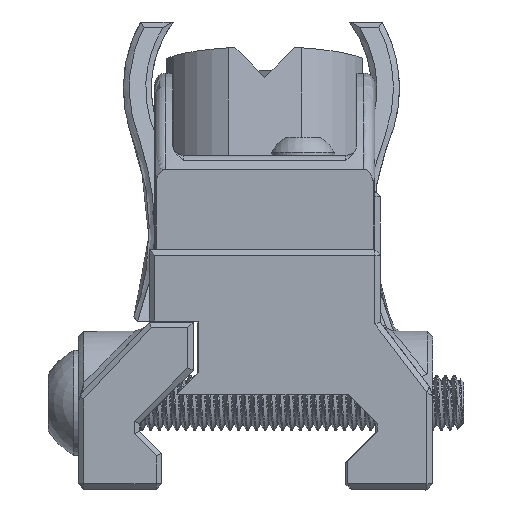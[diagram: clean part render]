
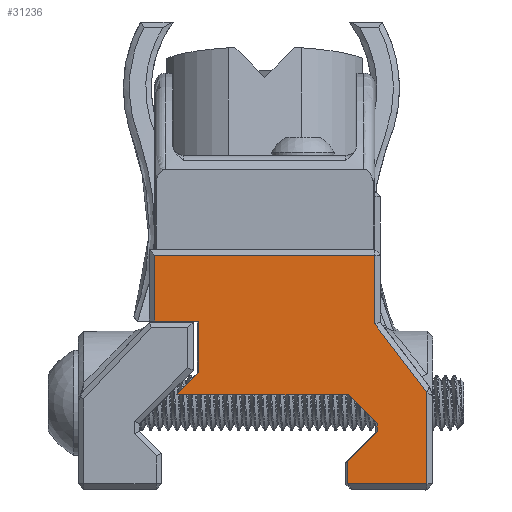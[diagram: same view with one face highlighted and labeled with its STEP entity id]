
A CAD part, front view. The second image highlights one B-rep face of the part: STEP entity #31236.
In plain terms, the highlighted planar face has unit normal (0, -1, 0).
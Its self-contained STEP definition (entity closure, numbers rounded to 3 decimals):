
#1353=PLANE('',#33986);
#4841=FACE_OUTER_BOUND('',#6821,.T.);
#6821=EDGE_LOOP('',(#26321,#26322,#26323,#26324,#26325,#26326,#26327,#26328,
#26329,#26330,#26331,#26332,#26333,#26334));
#8676=LINE('',#80153,#10592);
#8693=LINE('',#80186,#10609);
#8699=LINE('',#80198,#10615);
#8700=LINE('',#80201,#10616);
#8707=LINE('',#80217,#10623);
#8709=LINE('',#80220,#10625);
#8712=LINE('',#80224,#10628);
#8737=LINE('',#80277,#10653);
#8738=LINE('',#80279,#10654);
#8739=LINE('',#80281,#10655);
#8740=LINE('',#80283,#10656);
#8741=LINE('',#80284,#10657);
#8742=LINE('',#80286,#10658);
#8743=LINE('',#80287,#10659);
#10592=VECTOR('',#39924,10.);
#10609=VECTOR('',#39953,10.);
#10615=VECTOR('',#39967,10.);
#10616=VECTOR('',#39970,10.);
#10623=VECTOR('',#39981,10.);
#10625=VECTOR('',#39985,10.);
#10628=VECTOR('',#39990,10.);
#10653=VECTOR('',#40043,10.);
#10654=VECTOR('',#40044,10.);
#10655=VECTOR('',#40045,10.);
#10656=VECTOR('',#40046,10.);
#10657=VECTOR('',#40047,10.);
#10658=VECTOR('',#40048,10.);
#10659=VECTOR('',#40049,10.);
#14172=VERTEX_POINT('',#80150);
#14173=VERTEX_POINT('',#80152);
#14178=VERTEX_POINT('',#80167);
#14182=VERTEX_POINT('',#80179);
#14185=VERTEX_POINT('',#80194);
#14186=VERTEX_POINT('',#80200);
#14189=VERTEX_POINT('',#80207);
#14192=VERTEX_POINT('',#80214);
#14193=VERTEX_POINT('',#80216);
#14207=VERTEX_POINT('',#80276);
#14208=VERTEX_POINT('',#80278);
#14209=VERTEX_POINT('',#80280);
#14210=VERTEX_POINT('',#80282);
#14211=VERTEX_POINT('',#80285);
#18333=EDGE_CURVE('',#14172,#14173,#8676,.T.);
#18350=EDGE_CURVE('',#14182,#14178,#8693,.T.);
#18356=EDGE_CURVE('',#14185,#14182,#8699,.T.);
#18357=EDGE_CURVE('',#14186,#14185,#8700,.T.);
#18364=EDGE_CURVE('',#14192,#14193,#8707,.T.);
#18366=EDGE_CURVE('',#14193,#14189,#8709,.T.);
#18369=EDGE_CURVE('',#14189,#14186,#8712,.T.);
#18396=EDGE_CURVE('',#14192,#14207,#8737,.T.);
#18397=EDGE_CURVE('',#14207,#14208,#8738,.T.);
#18398=EDGE_CURVE('',#14208,#14209,#8739,.T.);
#18399=EDGE_CURVE('',#14210,#14209,#8740,.T.);
#18400=EDGE_CURVE('',#14173,#14210,#8741,.T.);
#18401=EDGE_CURVE('',#14211,#14172,#8742,.T.);
#18402=EDGE_CURVE('',#14178,#14211,#8743,.T.);
#26321=ORIENTED_EDGE('',*,*,#18350,.F.);
#26322=ORIENTED_EDGE('',*,*,#18356,.F.);
#26323=ORIENTED_EDGE('',*,*,#18357,.F.);
#26324=ORIENTED_EDGE('',*,*,#18369,.F.);
#26325=ORIENTED_EDGE('',*,*,#18366,.F.);
#26326=ORIENTED_EDGE('',*,*,#18364,.F.);
#26327=ORIENTED_EDGE('',*,*,#18396,.T.);
#26328=ORIENTED_EDGE('',*,*,#18397,.T.);
#26329=ORIENTED_EDGE('',*,*,#18398,.T.);
#26330=ORIENTED_EDGE('',*,*,#18399,.F.);
#26331=ORIENTED_EDGE('',*,*,#18400,.F.);
#26332=ORIENTED_EDGE('',*,*,#18333,.F.);
#26333=ORIENTED_EDGE('',*,*,#18401,.F.);
#26334=ORIENTED_EDGE('',*,*,#18402,.F.);
#31236=ADVANCED_FACE('',(#4841),#1353,.T.);
#33986=AXIS2_PLACEMENT_3D('',#80275,#40041,#40042);
#39924=DIRECTION('',(0.,0.,1.));
#39953=DIRECTION('',(-1.,0.,0.));
#39967=DIRECTION('',(0.,0.,-1.));
#39970=DIRECTION('',(0.605,0.,-0.796));
#39981=DIRECTION('',(0.,0.,1.));
#39985=DIRECTION('',(1.,0.,0.));
#39990=DIRECTION('',(0.,0.,-1.));
#40041=DIRECTION('center_axis',(0.,-1.,
0.));
#40042=DIRECTION('ref_axis',(-1.,0.,0.));
#40043=DIRECTION('',(1.,0.,0.));
#40044=DIRECTION('',(0.,0.,-1.));
#40045=DIRECTION('',(-0.707,0.,-0.707));
#40046=DIRECTION('',(-1.,0.,0.));
#40047=DIRECTION('',(-0.707,0.,0.707));
#40048=DIRECTION('',(0.707,0.,0.707));
#40049=DIRECTION('',(0.,0.,1.));
#80150=CARTESIAN_POINT('',(-57.745,-398.93,5.658));
#80152=CARTESIAN_POINT('',(-57.745,-398.93,6.363));
#80153=CARTESIAN_POINT('',(-57.745,-398.93,5.658));
#80167=CARTESIAN_POINT('',(-60.475,-398.929,0.91));
#80179=CARTESIAN_POINT('',(-53.245,-398.93,0.91));
#80186=CARTESIAN_POINT('',(-51.944,-398.93,0.91));
#80194=CARTESIAN_POINT('',(-53.245,-398.93,9.188));
#80198=CARTESIAN_POINT('',(-53.245,-398.93,20.715));
#80200=CARTESIAN_POINT('',(-57.981,-398.93,15.418));
#80201=CARTESIAN_POINT('',(-60.476,-398.929,18.7));
#80207=CARTESIAN_POINT('',(-57.981,-398.93,21.662));
#80214=CARTESIAN_POINT('',(-77.981,-398.926,15.686));
#80216=CARTESIAN_POINT('',(-77.981,-398.926,21.662));
#80217=CARTESIAN_POINT('',(-77.981,-398.926,19.768));
#80220=CARTESIAN_POINT('',(-64.812,-398.928,21.662));
#80224=CARTESIAN_POINT('',(-57.981,-398.93,28.308));
#80275=CARTESIAN_POINT('Origin',(-51.143,-398.931,32.074));
#80276=CARTESIAN_POINT('',(-73.981,-398.927,15.686));
#80277=CARTESIAN_POINT('',(-64.812,-398.928,15.686));
#80278=CARTESIAN_POINT('',(-73.981,-398.927,11.02));
#80279=CARTESIAN_POINT('',(-73.981,-398.927,23.88));
#80280=CARTESIAN_POINT('',(-75.99,-398.927,9.01));
#80281=CARTESIAN_POINT('',(-63.008,-398.929,21.993));
#80282=CARTESIAN_POINT('',(-60.392,-398.929,9.01));
#80283=CARTESIAN_POINT('',(-51.143,-398.931,9.01));
#80284=CARTESIAN_POINT('',(-57.745,-398.93,6.363));
#80285=CARTESIAN_POINT('',(-60.475,-398.929,2.928));
#80286=CARTESIAN_POINT('',(-60.475,-398.929,2.928));
#80287=CARTESIAN_POINT('',(-60.475,-398.929,0.41));
